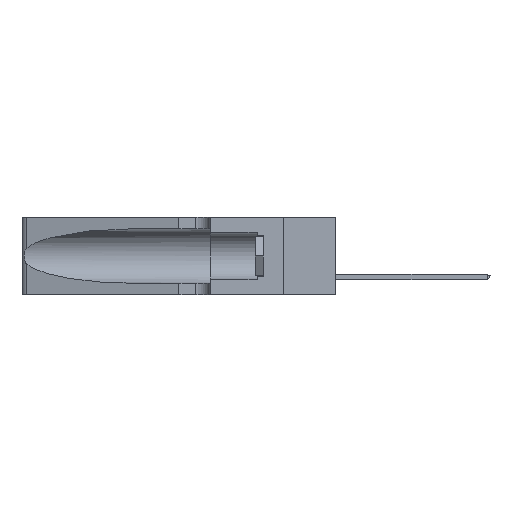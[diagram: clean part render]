
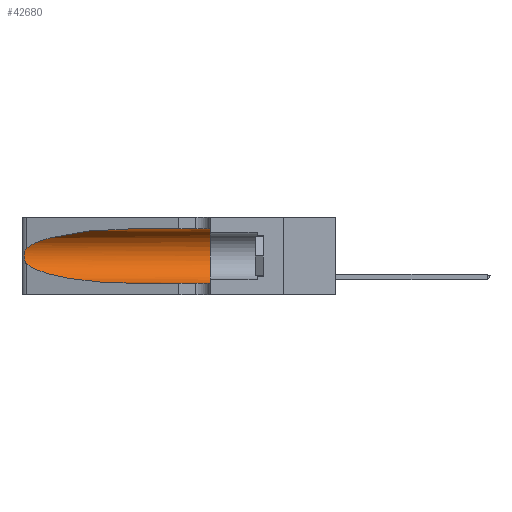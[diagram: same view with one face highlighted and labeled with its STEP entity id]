
A CAD part, left-side view. The second image highlights one B-rep face of the part: STEP entity #42680.
In plain terms, the highlighted cylindrical face has radius 3.308 mm (diameter 6.617 mm), a partial arc.
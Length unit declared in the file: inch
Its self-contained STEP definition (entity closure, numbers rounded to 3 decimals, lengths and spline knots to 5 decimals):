
#365 = CARTESIAN_POINT ( 'NONE',  ( 0.25487, 1.22718, 0.14631 ) ) ;
#745 = ORIENTED_EDGE ( 'NONE', *, *, #3949, .T. ) ;
#779 = AXIS2_PLACEMENT_3D ( 'NONE', #45091, #37709, #37560 ) ;
#1284 = CARTESIAN_POINT ( 'NONE',  ( 0.1305, 1.61858, 0.05475 ) ) ;
#1466 = CARTESIAN_POINT ( 'NONE',  ( 0.1305, 0.35, 0.05475 ) ) ;
#2261 = VERTEX_POINT ( 'NONE', #1466 ) ;
#3133 = VERTEX_POINT ( 'NONE', #12959 ) ;
#3292 = AXIS2_PLACEMENT_3D ( 'NONE', #6772, #14109, #34591 ) ;
#3402 = CARTESIAN_POINT ( 'NONE',  ( 0.1305, 0.72297, 0.05475 ) ) ;
#3406 = CARTESIAN_POINT ( 'NONE',  ( 0.25787, 1.23484, 0.2124 ) ) ;
#3949 = EDGE_CURVE ( 'NONE', #37958, #15589, #34219, .T. ) ;
#5141 = CARTESIAN_POINT ( 'NONE',  ( 0.25555, 1.22994, 0.2215 ) ) ;
#5462 = CARTESIAN_POINT ( 'NONE',  ( 0.1305, 0.72297, 0.31525 ) ) ;
#5881 = VECTOR ( 'NONE', #43566, 39.37008 ) ;
#6422 = CARTESIAN_POINT ( 'NONE',  ( 0.1305, 0.72297, 0.31525 ) ) ;
#6772 = CARTESIAN_POINT ( 'NONE',  ( 0.1305, 1.61858, 0.185 ) ) ;
#8609 = LINE ( 'NONE', #1284, #5881 ) ;
#9121 = DIRECTION ( 'NONE',  ( 0., -1., 0. ) ) ;
#9803 = CARTESIAN_POINT ( 'NONE',  ( 0.26075, 1.23896, 0.19203 ) ) ;
#10094 = CARTESIAN_POINT ( 'NONE',  ( 0.25487, 1.22718, 0.22369 ) ) ;
#10614 = CARTESIAN_POINT ( 'NONE',  ( 0.25487, 1.22718, 0.14631 ) ) ;
#10975 = ORIENTED_EDGE ( 'NONE', *, *, #38072, .F. ) ;
#11052 = CARTESIAN_POINT ( 'NONE',  ( 0.2373, 1.15595, 0.08982 ) ) ;
#12959 = CARTESIAN_POINT ( 'NONE',  ( 0.25487, 1.22718, 0.14631 ) ) ;
#14109 = DIRECTION ( 'NONE',  ( 0., -1., 0. ) ) ;
#14232 = ORIENTED_EDGE ( 'NONE', *, *, #19732, .T. ) ;
#14766 = CYLINDRICAL_SURFACE ( 'NONE', #3292, 0.13025 ) ;
#15407 = CARTESIAN_POINT ( 'NONE',  ( 0.26075, 1.23896, 0.178 ) ) ;
#15589 = VERTEX_POINT ( 'NONE', #43863 ) ;
#16973 = CARTESIAN_POINT ( 'NONE',  ( 0.2373, 1.15595, 0.28018 ) ) ;
#17281 = CARTESIAN_POINT ( 'NONE',  ( 0.25789, 1.23486, 0.15765 ) ) ;
#17493 = CARTESIAN_POINT ( 'NONE',  ( 0.18966, 0.96281, 0.05475 ) ) ;
#18879 = CARTESIAN_POINT ( 'NONE',  ( 0.25487, 1.22718, 0.22369 ) ) ;
#19477 = CARTESIAN_POINT ( 'NONE',  ( 0.1305, 1.61858, 0.31525 ) ) ;
#19732 = EDGE_CURVE ( 'NONE', #15589, #3133, #25370, .T. ) ;
#19942 = VECTOR ( 'NONE', #9121, 39.37008 ) ;
#20097 = EDGE_CURVE ( 'NONE', #37958, #35994, #33735, .T. ) ;
#20502 = VERTEX_POINT ( 'NONE', #3402 ) ;
#21446 = CARTESIAN_POINT ( 'NONE',  ( 0.1305, 0.72297, 0.05475 ) ) ;
#21993 =( BOUNDED_CURVE ( )  B_SPLINE_CURVE ( 3, ( #10614, #11052, #17493, #21446 ),
 .UNSPECIFIED., .F., .T. ) 
 B_SPLINE_CURVE_WITH_KNOTS ( ( 4, 4 ),
 ( 3.44316, 4.71239 ),
 .UNSPECIFIED. ) 
 CURVE ( )  GEOMETRIC_REPRESENTATION_ITEM ( )  RATIONAL_B_SPLINE_CURVE ( ( 1., 0.87, 0.87, 1. ) ) 
 REPRESENTATION_ITEM ( '' )  );
#22008 = CARTESIAN_POINT ( 'NONE',  ( 0.25854, 1.2359, 0.20912 ) ) ;
#22020 = CARTESIAN_POINT ( 'NONE',  ( 0.1305, 0.35, 0.31525 ) ) ;
#22175 = CIRCLE ( 'NONE', #779, 0.13025 ) ;
#23368 = ORIENTED_EDGE ( 'NONE', *, *, #44009, .T. ) ;
#23524 = CARTESIAN_POINT ( 'NONE',  ( 0.26018, 1.23835, 0.19895 ) ) ;
#25370 = B_SPLINE_CURVE_WITH_KNOTS ( 'NONE', 3,
 ( #18879, #5141, #26384, #3406, #22008, #23524, #9803, #15407, #25691, #25532, #17281, #37442, #31183, #365 ),
 .UNSPECIFIED., .F., .F.,
 ( 4, 2, 2, 2, 2, 2, 4 ),
 ( 0., 0.00027, 0.00053, 0.00107, 0.0016, 0.00187, 0.00214 ),
 .UNSPECIFIED. ) ;
#25532 = CARTESIAN_POINT ( 'NONE',  ( 0.25856, 1.23593, 0.16098 ) ) ;
#25691 = CARTESIAN_POINT ( 'NONE',  ( 0.26017, 1.23833, 0.17102 ) ) ;
#26384 = CARTESIAN_POINT ( 'NONE',  ( 0.25639, 1.23184, 0.21858 ) ) ;
#27885 = EDGE_CURVE ( 'NONE', #3133, #20502, #21993, .T. ) ;
#28673 = ORIENTED_EDGE ( 'NONE', *, *, #27885, .T. ) ;
#30652 = CARTESIAN_POINT ( 'NONE',  ( 0.18966, 0.96281, 0.31525 ) ) ;
#31183 = CARTESIAN_POINT ( 'NONE',  ( 0.25555, 1.22993, 0.14849 ) ) ;
#33735 = LINE ( 'NONE', #19477, #19942 ) ;
#34219 =( BOUNDED_CURVE ( )  B_SPLINE_CURVE ( 3, ( #6422, #30652, #16973, #10094 ),
 .UNSPECIFIED., .F., .T. ) 
 B_SPLINE_CURVE_WITH_KNOTS ( ( 4, 4 ),
 ( 1.5708, 2.84003 ),
 .UNSPECIFIED. ) 
 CURVE ( )  GEOMETRIC_REPRESENTATION_ITEM ( )  RATIONAL_B_SPLINE_CURVE ( ( 1., 0.87, 0.87, 1. ) ) 
 REPRESENTATION_ITEM ( '' )  );
#34591 = DIRECTION ( 'NONE',  ( 0., 0., -1. ) ) ;
#35994 = VERTEX_POINT ( 'NONE', #22020 ) ;
#37442 = CARTESIAN_POINT ( 'NONE',  ( 0.25639, 1.23186, 0.15144 ) ) ;
#37560 = DIRECTION ( 'NONE',  ( 0., 0., 1. ) ) ;
#37709 = DIRECTION ( 'NONE',  ( 0., 1., 0. ) ) ;
#37958 = VERTEX_POINT ( 'NONE', #5462 ) ;
#38072 = EDGE_CURVE ( 'NONE', #35994, #2261, #22175, .T. ) ;
#39444 = EDGE_LOOP ( 'NONE', ( #745, #14232, #28673, #23368, #10975, #44399 ) ) ;
#42680 = ADVANCED_FACE ( 'NONE', ( #42904 ), #14766, .F. ) ;
#42904 = FACE_OUTER_BOUND ( 'NONE', #39444, .T. ) ;
#43566 = DIRECTION ( 'NONE',  ( 0., -1., 0. ) ) ;
#43863 = CARTESIAN_POINT ( 'NONE',  ( 0.25487, 1.22718, 0.22369 ) ) ;
#44009 = EDGE_CURVE ( 'NONE', #20502, #2261, #8609, .T. ) ;
#44399 = ORIENTED_EDGE ( 'NONE', *, *, #20097, .F. ) ;
#45091 = CARTESIAN_POINT ( 'NONE',  ( 0.1305, 0.35, 0.185 ) ) ;
